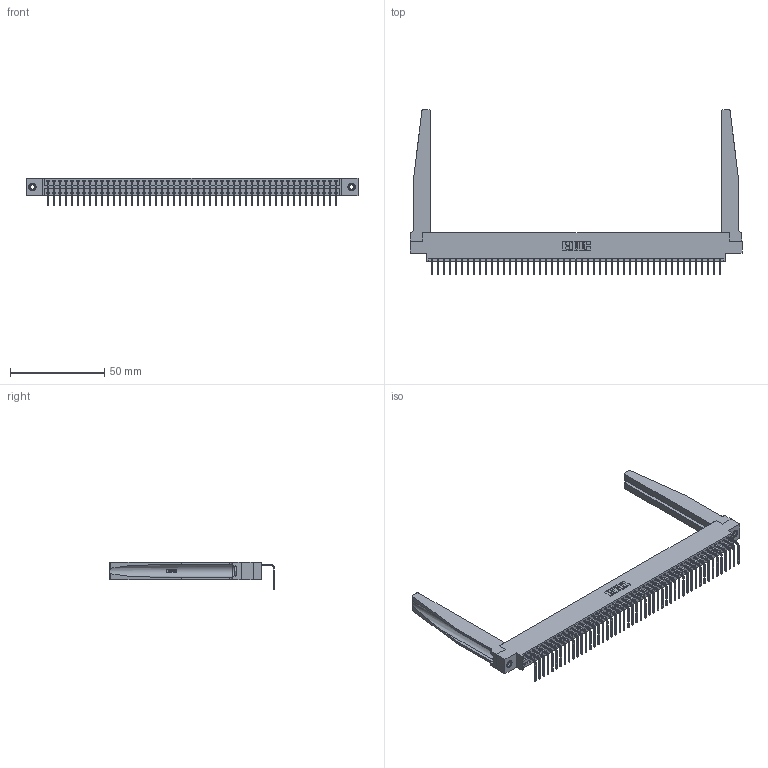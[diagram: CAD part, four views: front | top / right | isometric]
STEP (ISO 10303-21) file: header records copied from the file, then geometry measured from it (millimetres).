
FILE_DESCRIPTION (( 'STEP AP203' ), '1' );
FILE_NAME ('396-049-558-678.STEP', '2019-11-01T08:38:14', ( '' ), ( '' ), 'SwSTEP 2.0', 'SolidWorks 2016', '' );
FILE_SCHEMA (( 'CONFIG_CONTROL_DESIGN' ));
Length unit declared in the file: inch
Products named in the file (5): 346 Part_0.170 Offset - 0.156 Dia-TH; 345-292-001_558 Tail - 2; 346-220-078_345-220-078; 345-250-001_345-250-001-102; 396-049-558-678
Assembly tree (54 placements, depth 2):
  396-049-558-678
    346 Part_0.170 Offset - 0.156 Dia-TH
    345-292-001_558 Tail - 2  x49
    346-220-078_345-220-078  x2
    345-250-001_345-250-001-102  x2
Bounding box: 176.15 x 87.44 x 14.73 mm (x, y, z)
Volume: 23827.1 mm3; surface area: 28895.5 mm2
Topology: 54 solids, 54 shells, 3300 faces, 9867 edges, 6502 vertices
Faces by surface type: plane 2280, cylinder 968, bspline 36, cone 12, torus 4
Entity records: 34432 total; most frequent: CARTESIAN_POINT 6814, ORIENTED_EDGE 5686, DIRECTION 4987, EDGE_CURVE 2843, LINE 2421, VECTOR 2421, VERTEX_POINT 1888, AXIS2_PLACEMENT_3D 1283
